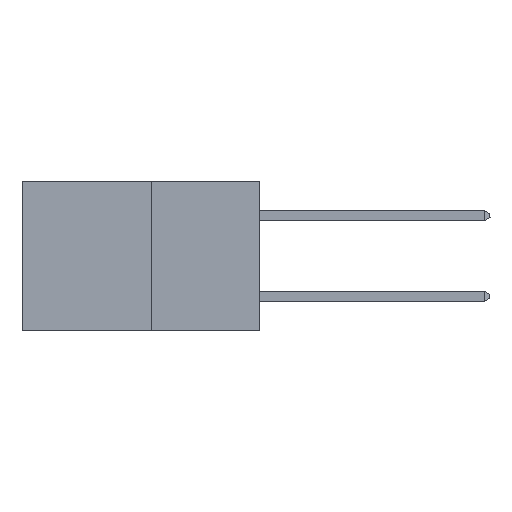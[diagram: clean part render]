
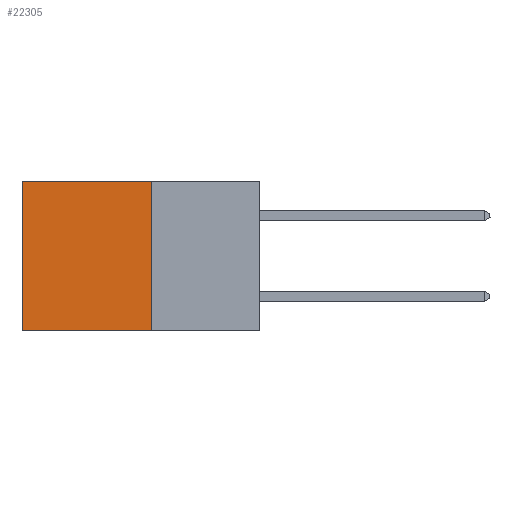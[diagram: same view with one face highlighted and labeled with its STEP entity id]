
A CAD part, left-side view. The second image highlights one B-rep face of the part: STEP entity #22305.
In plain terms, the highlighted planar face has unit normal (-1, 0, 0).
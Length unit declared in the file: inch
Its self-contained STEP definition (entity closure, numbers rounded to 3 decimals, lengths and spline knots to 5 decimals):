
#1056 = ORIENTED_EDGE ( 'NONE', *, *, #20326, .T. ) ;
#1758 = AXIS2_PLACEMENT_3D ( 'NONE', #20860, #17249, #11859 ) ;
#2060 = CARTESIAN_POINT ( 'NONE',  ( 0.277, 0.27, 0. ) ) ;
#2240 = VECTOR ( 'NONE', #4405, 39.37008 ) ;
#2582 = EDGE_CURVE ( 'NONE', #15231, #21478, #8072, .T. ) ;
#3111 = EDGE_CURVE ( 'NONE', #21478, #7618, #15991, .T. ) ;
#3124 = CARTESIAN_POINT ( 'NONE',  ( 0.277, 0.27, 0. ) ) ;
#3671 = DIRECTION ( 'NONE',  ( 0., 1., 0. ) ) ;
#4405 = DIRECTION ( 'NONE',  ( 0., 0., -1. ) ) ;
#4592 = VERTEX_POINT ( 'NONE', #22020 ) ;
#7618 = VERTEX_POINT ( 'NONE', #9220 ) ;
#7715 = CARTESIAN_POINT ( 'NONE',  ( 0.277, 0.27, -0.37 ) ) ;
#8072 = LINE ( 'NONE', #17149, #21915 ) ;
#9220 = CARTESIAN_POINT ( 'NONE',  ( 0.277, 0.59, -0.37 ) ) ;
#10601 = VECTOR ( 'NONE', #3671, 39.37008 ) ;
#11415 = LINE ( 'NONE', #13591, #2240 ) ;
#11859 = DIRECTION ( 'NONE',  ( 0., 0., -1. ) ) ;
#12042 = VECTOR ( 'NONE', #20297, 39.37008 ) ;
#13591 = CARTESIAN_POINT ( 'NONE',  ( 0.277, 0.59, -0.37 ) ) ;
#14827 = CARTESIAN_POINT ( 'NONE',  ( 0.277, 0.27, -0.37 ) ) ;
#15140 = ORIENTED_EDGE ( 'NONE', *, *, #3111, .F. ) ;
#15231 = VERTEX_POINT ( 'NONE', #3124 ) ;
#15508 = EDGE_CURVE ( 'NONE', #15231, #4592, #16881, .T. ) ;
#15991 = LINE ( 'NONE', #7715, #10601 ) ;
#16881 = LINE ( 'NONE', #2060, #12042 ) ;
#17045 = DIRECTION ( 'NONE',  ( 0., 0., -1. ) ) ;
#17149 = CARTESIAN_POINT ( 'NONE',  ( 0.277, 0.27, -0.37 ) ) ;
#17249 = DIRECTION ( 'NONE',  ( 1., 0., 0. ) ) ;
#19417 = EDGE_LOOP ( 'NONE', ( #1056, #15140, #20674, #21074 ) ) ;
#20297 = DIRECTION ( 'NONE',  ( 0., 1., 0. ) ) ;
#20326 = EDGE_CURVE ( 'NONE', #4592, #7618, #11415, .T. ) ;
#20674 = ORIENTED_EDGE ( 'NONE', *, *, #2582, .F. ) ;
#20860 = CARTESIAN_POINT ( 'NONE',  ( 0.277, 0.27, -0.37 ) ) ;
#21074 = ORIENTED_EDGE ( 'NONE', *, *, #15508, .T. ) ;
#21209 = FACE_OUTER_BOUND ( 'NONE', #19417, .T. ) ;
#21478 = VERTEX_POINT ( 'NONE', #14827 ) ;
#21915 = VECTOR ( 'NONE', #17045, 39.37008 ) ;
#22020 = CARTESIAN_POINT ( 'NONE',  ( 0.277, 0.59, 0. ) ) ;
#22305 = ADVANCED_FACE ( 'NONE', ( #21209 ), #22648, .F. ) ;
#22648 = PLANE ( 'NONE',  #1758 ) ;
